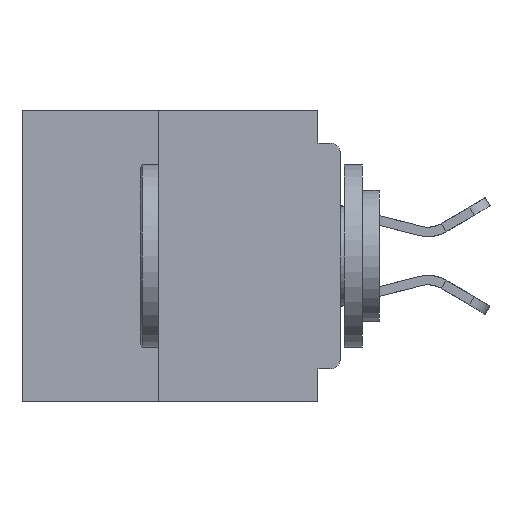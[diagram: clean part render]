
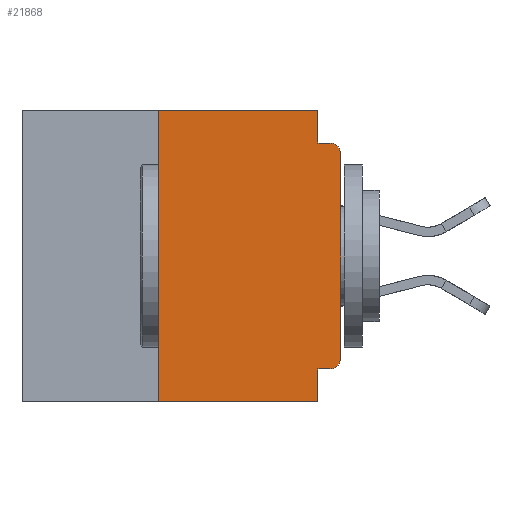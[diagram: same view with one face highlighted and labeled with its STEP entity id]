
A CAD part, left-side view. The second image highlights one B-rep face of the part: STEP entity #21868.
In plain terms, the highlighted planar face has unit normal (-1, 0, 0).
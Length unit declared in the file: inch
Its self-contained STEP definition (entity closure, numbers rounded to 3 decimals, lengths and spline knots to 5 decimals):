
#2241 = ORIENTED_EDGE ( 'NONE', *, *, #3329, .F. ) ;
#2621 = LINE ( 'NONE', #10799, #13521 ) ;
#3329 = EDGE_CURVE ( 'NONE', #45285, #36200, #6985, .T. ) ;
#4011 = EDGE_CURVE ( 'NONE', #12254, #36639, #43831, .T. ) ;
#4313 = CARTESIAN_POINT ( 'NONE',  ( 0., 0.031, -0.355 ) ) ;
#4761 = VERTEX_POINT ( 'NONE', #19548 ) ;
#5778 = ORIENTED_EDGE ( 'NONE', *, *, #23261, .T. ) ;
#5967 = DIRECTION ( 'NONE',  ( 0., 0., 1. ) ) ;
#6964 = ORIENTED_EDGE ( 'NONE', *, *, #46677, .T. ) ;
#6985 = LINE ( 'NONE', #27308, #46674 ) ;
#7437 = ORIENTED_EDGE ( 'NONE', *, *, #38790, .F. ) ;
#7602 = DIRECTION ( 'NONE',  ( -1., 0., 0. ) ) ;
#8166 = CARTESIAN_POINT ( 'NONE',  ( 0., 0.031, -0.045 ) ) ;
#8837 = EDGE_CURVE ( 'NONE', #29038, #29817, #46126, .T. ) ;
#9395 = VECTOR ( 'NONE', #5967, 39.37008 ) ;
#9736 = DIRECTION ( 'NONE',  ( 0., 1., 0. ) ) ;
#10548 = LINE ( 'NONE', #24096, #9395 ) ;
#10799 = CARTESIAN_POINT ( 'NONE',  ( 0., 0.25, -0.4 ) ) ;
#12239 = VECTOR ( 'NONE', #36000, 39.37008 ) ;
#12254 = VERTEX_POINT ( 'NONE', #39607 ) ;
#13181 = CARTESIAN_POINT ( 'NONE',  ( 0., 0.25, 0. ) ) ;
#13363 = DIRECTION ( 'NONE',  ( 0., -1., 0. ) ) ;
#13383 = VECTOR ( 'NONE', #9736, 39.37008 ) ;
#13521 = VECTOR ( 'NONE', #36228, 39.37008 ) ;
#14511 = ORIENTED_EDGE ( 'NONE', *, *, #40114, .T. ) ;
#15487 = EDGE_CURVE ( 'NONE', #12254, #45285, #23041, .T. ) ;
#16788 = VECTOR ( 'NONE', #24427, 39.37008 ) ;
#16950 = ORIENTED_EDGE ( 'NONE', *, *, #8837, .F. ) ;
#17092 = CIRCLE ( 'NONE', #24921, 0.015 ) ;
#17724 = FACE_OUTER_BOUND ( 'NONE', #26551, .T. ) ;
#18921 = VERTEX_POINT ( 'NONE', #41448 ) ;
#19548 = CARTESIAN_POINT ( 'NONE',  ( 0., 0.25, -0.4 ) ) ;
#19747 = DIRECTION ( 'NONE',  ( 0., 0., -1. ) ) ;
#19854 = DIRECTION ( 'NONE',  ( -1., 0., 0. ) ) ;
#20011 = CARTESIAN_POINT ( 'NONE',  ( 0., 0.015, -0.34 ) ) ;
#21246 = CARTESIAN_POINT ( 'NONE',  ( 0., 0.031, -0.4 ) ) ;
#21420 = CARTESIAN_POINT ( 'NONE',  ( 0., 0.437, -0.4 ) ) ;
#21868 = ADVANCED_FACE ( 'NONE', ( #17724 ), #42196, .F. ) ;
#23041 = LINE ( 'NONE', #24363, #13383 ) ;
#23261 = EDGE_CURVE ( 'NONE', #18921, #45878, #17092, .T. ) ;
#24096 = CARTESIAN_POINT ( 'NONE',  ( 0., 0., 0. ) ) ;
#24109 = DIRECTION ( 'NONE',  ( 0., 0., -1. ) ) ;
#24127 = CARTESIAN_POINT ( 'NONE',  ( 0., 0.437, 0. ) ) ;
#24363 = CARTESIAN_POINT ( 'NONE',  ( 0., 0., -0.355 ) ) ;
#24427 = DIRECTION ( 'NONE',  ( 0., -1., 0. ) ) ;
#24583 = AXIS2_PLACEMENT_3D ( 'NONE', #31277, #45763, #24109 ) ;
#24921 = AXIS2_PLACEMENT_3D ( 'NONE', #29381, #7602, #33040 ) ;
#26152 = AXIS2_PLACEMENT_3D ( 'NONE', #20011, #19854, #19747 ) ;
#26551 = EDGE_LOOP ( 'NONE', ( #6964, #5778, #40848, #16950, #31463, #7437, #14511, #2241, #42887, #36584 ) ) ;
#26689 = VECTOR ( 'NONE', #13363, 39.37008 ) ;
#27308 = CARTESIAN_POINT ( 'NONE',  ( 0., 0.031, -0.4 ) ) ;
#27767 = DIRECTION ( 'NONE',  ( 0., 0., -1. ) ) ;
#27812 = LINE ( 'NONE', #24127, #26689 ) ;
#29038 = VERTEX_POINT ( 'NONE', #42983 ) ;
#29381 = CARTESIAN_POINT ( 'NONE',  ( 0., 0.015, -0.06 ) ) ;
#29761 = CARTESIAN_POINT ( 'NONE',  ( 0., 0.015, -0.045 ) ) ;
#29817 = VERTEX_POINT ( 'NONE', #8166 ) ;
#31277 = CARTESIAN_POINT ( 'NONE',  ( 0., 0.437, 0. ) ) ;
#31463 = ORIENTED_EDGE ( 'NONE', *, *, #33606, .F. ) ;
#31552 = LINE ( 'NONE', #21420, #12239 ) ;
#33040 = DIRECTION ( 'NONE',  ( 0., 0., -1. ) ) ;
#33606 = EDGE_CURVE ( 'NONE', #41732, #29038, #27812, .T. ) ;
#36000 = DIRECTION ( 'NONE',  ( 0., -1., 0. ) ) ;
#36200 = VERTEX_POINT ( 'NONE', #21246 ) ;
#36228 = DIRECTION ( 'NONE',  ( 0., 0., 1. ) ) ;
#36584 = ORIENTED_EDGE ( 'NONE', *, *, #4011, .T. ) ;
#36607 = VECTOR ( 'NONE', #42696, 39.37008 ) ;
#36639 = VERTEX_POINT ( 'NONE', #37869 ) ;
#37350 = EDGE_CURVE ( 'NONE', #29817, #45878, #45610, .T. ) ;
#37869 = CARTESIAN_POINT ( 'NONE',  ( 0., 0., -0.34 ) ) ;
#38790 = EDGE_CURVE ( 'NONE', #4761, #41732, #2621, .T. ) ;
#39607 = CARTESIAN_POINT ( 'NONE',  ( 0., 0.015, -0.355 ) ) ;
#40114 = EDGE_CURVE ( 'NONE', #4761, #36200, #31552, .T. ) ;
#40848 = ORIENTED_EDGE ( 'NONE', *, *, #37350, .F. ) ;
#41448 = CARTESIAN_POINT ( 'NONE',  ( 0., 0., -0.06 ) ) ;
#41732 = VERTEX_POINT ( 'NONE', #13181 ) ;
#42196 = PLANE ( 'NONE',  #24583 ) ;
#42524 = CARTESIAN_POINT ( 'NONE',  ( 0., 0., -0.045 ) ) ;
#42696 = DIRECTION ( 'NONE',  ( 0., 0., -1. ) ) ;
#42887 = ORIENTED_EDGE ( 'NONE', *, *, #15487, .F. ) ;
#42983 = CARTESIAN_POINT ( 'NONE',  ( 0., 0.031, 0. ) ) ;
#43831 = CIRCLE ( 'NONE', #26152, 0.015 ) ;
#45285 = VERTEX_POINT ( 'NONE', #4313 ) ;
#45610 = LINE ( 'NONE', #42524, #16788 ) ;
#45763 = DIRECTION ( 'NONE',  ( 1., 0., 0. ) ) ;
#45878 = VERTEX_POINT ( 'NONE', #29761 ) ;
#46123 = CARTESIAN_POINT ( 'NONE',  ( 0., 0.031, 0. ) ) ;
#46126 = LINE ( 'NONE', #46123, #36607 ) ;
#46674 = VECTOR ( 'NONE', #27767, 39.37008 ) ;
#46677 = EDGE_CURVE ( 'NONE', #36639, #18921, #10548, .T. ) ;
